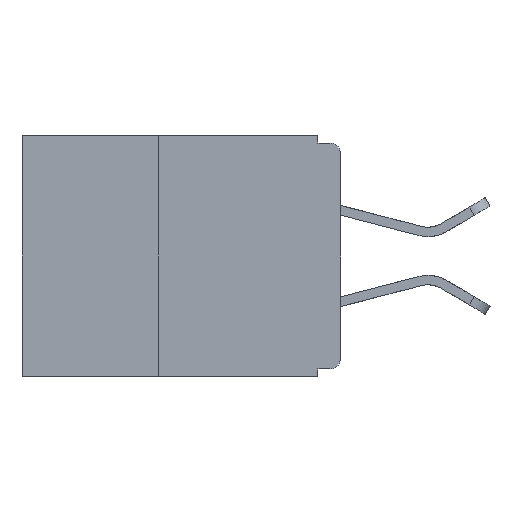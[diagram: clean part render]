
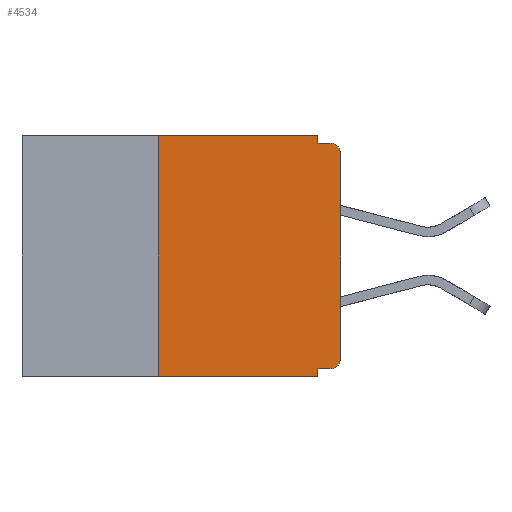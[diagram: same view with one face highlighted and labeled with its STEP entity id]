
A CAD part, left-side view. The second image highlights one B-rep face of the part: STEP entity #4534.
In plain terms, the highlighted planar face has unit normal (-1, 0, 0).
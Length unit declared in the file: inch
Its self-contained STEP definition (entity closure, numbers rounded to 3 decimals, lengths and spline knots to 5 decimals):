
#111 = CARTESIAN_POINT ( 'NONE',  ( 0., 0.031, 0. ) ) ;
#301 = CARTESIAN_POINT ( 'NONE',  ( 0., 0., -0.32 ) ) ;
#302 = CARTESIAN_POINT ( 'NONE',  ( 0., 0., -0.025 ) ) ;
#373 = DIRECTION ( 'NONE',  ( 0., 1., 0. ) ) ;
#602 = DIRECTION ( 'NONE',  ( 0., 0., -1. ) ) ;
#776 = VERTEX_POINT ( 'NONE', #18537 ) ;
#966 = CARTESIAN_POINT ( 'NONE',  ( 0., 0.031, -0.33 ) ) ;
#1257 = DIRECTION ( 'NONE',  ( -1., 0., 0. ) ) ;
#1378 = EDGE_LOOP ( 'NONE', ( #11181, #12087, #12539, #12990, #17019, #17448, #14291, #17869, #10957, #3368 ) ) ;
#1664 = DIRECTION ( 'NONE',  ( 0., 0., -1. ) ) ;
#1683 = DIRECTION ( 'NONE',  ( -1., 0., 0. ) ) ;
#1689 = CARTESIAN_POINT ( 'NONE',  ( 0., 0.015, -0.025 ) ) ;
#1736 = AXIS2_PLACEMENT_3D ( 'NONE', #1835, #1257, #602 ) ;
#1835 = CARTESIAN_POINT ( 'NONE',  ( 0., 0.015, -0.305 ) ) ;
#2115 = VECTOR ( 'NONE', #15954, 39.37008 ) ;
#2539 = CARTESIAN_POINT ( 'NONE',  ( 0., 0.031, -0.32 ) ) ;
#2722 = VECTOR ( 'NONE', #5000, 39.37008 ) ;
#3055 = VERTEX_POINT ( 'NONE', #302 ) ;
#3368 = ORIENTED_EDGE ( 'NONE', *, *, #5415, .T. ) ;
#3526 = VECTOR ( 'NONE', #8269, 39.37008 ) ;
#3916 = VECTOR ( 'NONE', #11428, 39.37008 ) ;
#4034 = LINE ( 'NONE', #8231, #3526 ) ;
#4182 = AXIS2_PLACEMENT_3D ( 'NONE', #1689, #1683, #1664 ) ;
#4226 = CARTESIAN_POINT ( 'NONE',  ( 0., 0.015, -0.32 ) ) ;
#4534 = ADVANCED_FACE ( 'NONE', ( #9555 ), #14995, .F. ) ;
#4952 = CARTESIAN_POINT ( 'NONE',  ( 0., 0.437, -0.33 ) ) ;
#5000 = DIRECTION ( 'NONE',  ( 0., -1., 0. ) ) ;
#5022 = CARTESIAN_POINT ( 'NONE',  ( 0., 0., -0.01 ) ) ;
#5252 = VERTEX_POINT ( 'NONE', #111 ) ;
#5415 = EDGE_CURVE ( 'NONE', #12051, #15168, #18578, .T. ) ;
#5554 = CARTESIAN_POINT ( 'NONE',  ( 0., 0.25, -0.33 ) ) ;
#5567 = CARTESIAN_POINT ( 'NONE',  ( 0., 0., -0.305 ) ) ;
#5965 = CARTESIAN_POINT ( 'NONE',  ( 0., 0.031, 0. ) ) ;
#6213 = VECTOR ( 'NONE', #6571, 39.37008 ) ;
#6506 = VERTEX_POINT ( 'NONE', #966 ) ;
#6571 = DIRECTION ( 'NONE',  ( 0., -1., 0. ) ) ;
#6614 = LINE ( 'NONE', #16794, #17921 ) ;
#6854 = LINE ( 'NONE', #4952, #2722 ) ;
#8231 = CARTESIAN_POINT ( 'NONE',  ( 0., 0.031, -0.33 ) ) ;
#8269 = DIRECTION ( 'NONE',  ( 0., 0., -1. ) ) ;
#8357 = VERTEX_POINT ( 'NONE', #2539 ) ;
#8415 = EDGE_CURVE ( 'NONE', #3055, #16793, #11207, .T. ) ;
#9001 = VERTEX_POINT ( 'NONE', #10306 ) ;
#9039 = EDGE_CURVE ( 'NONE', #15168, #3055, #18685, .T. ) ;
#9431 = CARTESIAN_POINT ( 'NONE',  ( 0., 0., 0. ) ) ;
#9555 = FACE_OUTER_BOUND ( 'NONE', #1378, .T. ) ;
#10234 = LINE ( 'NONE', #5965, #2115 ) ;
#10306 = CARTESIAN_POINT ( 'NONE',  ( 0., 0.25, 0. ) ) ;
#10372 = DIRECTION ( 'NONE',  ( 0., 0., 1. ) ) ;
#10957 = ORIENTED_EDGE ( 'NONE', *, *, #11390, .F. ) ;
#11181 = ORIENTED_EDGE ( 'NONE', *, *, #9039, .T. ) ;
#11207 = CIRCLE ( 'NONE', #4182, 0.015 ) ;
#11390 = EDGE_CURVE ( 'NONE', #12051, #8357, #18850, .T. ) ;
#11428 = DIRECTION ( 'NONE',  ( 0., -1., 0. ) ) ;
#11862 = EDGE_CURVE ( 'NONE', #8357, #6506, #4034, .T. ) ;
#11908 = LINE ( 'NONE', #12014, #3916 ) ;
#12014 = CARTESIAN_POINT ( 'NONE',  ( 0., 0.437, 0. ) ) ;
#12051 = VERTEX_POINT ( 'NONE', #4226 ) ;
#12087 = ORIENTED_EDGE ( 'NONE', *, *, #8415, .T. ) ;
#12539 = ORIENTED_EDGE ( 'NONE', *, *, #17848, .F. ) ;
#12990 = ORIENTED_EDGE ( 'NONE', *, *, #16503, .F. ) ;
#13776 = EDGE_CURVE ( 'NONE', #18763, #6506, #6854, .T. ) ;
#14291 = ORIENTED_EDGE ( 'NONE', *, *, #13776, .T. ) ;
#14353 = EDGE_CURVE ( 'NONE', #9001, #5252, #11908, .T. ) ;
#14674 = EDGE_CURVE ( 'NONE', #18763, #9001, #6614, .T. ) ;
#14897 = DIRECTION ( 'NONE',  ( 0., 0., -1. ) ) ;
#14941 = DIRECTION ( 'NONE',  ( 1., 0., 0. ) ) ;
#14995 = PLANE ( 'NONE',  #18531 ) ;
#15168 = VERTEX_POINT ( 'NONE', #5567 ) ;
#15276 = VECTOR ( 'NONE', #373, 39.37008 ) ;
#15346 = CARTESIAN_POINT ( 'NONE',  ( 0., 0.015, -0.01 ) ) ;
#15526 = CARTESIAN_POINT ( 'NONE',  ( 0., 0.437, 0. ) ) ;
#15954 = DIRECTION ( 'NONE',  ( 0., 0., -1. ) ) ;
#16503 = EDGE_CURVE ( 'NONE', #5252, #776, #10234, .T. ) ;
#16793 = VERTEX_POINT ( 'NONE', #15346 ) ;
#16794 = CARTESIAN_POINT ( 'NONE',  ( 0., 0.25, -0.33 ) ) ;
#17019 = ORIENTED_EDGE ( 'NONE', *, *, #14353, .F. ) ;
#17051 = DIRECTION ( 'NONE',  ( 0., 0., 1. ) ) ;
#17448 = ORIENTED_EDGE ( 'NONE', *, *, #14674, .F. ) ;
#17561 = LINE ( 'NONE', #5022, #6213 ) ;
#17848 = EDGE_CURVE ( 'NONE', #776, #16793, #17561, .T. ) ;
#17869 = ORIENTED_EDGE ( 'NONE', *, *, #11862, .F. ) ;
#17921 = VECTOR ( 'NONE', #17051, 39.37008 ) ;
#18256 = VECTOR ( 'NONE', #10372, 39.37008 ) ;
#18531 = AXIS2_PLACEMENT_3D ( 'NONE', #15526, #14941, #14897 ) ;
#18537 = CARTESIAN_POINT ( 'NONE',  ( 0., 0.031, -0.01 ) ) ;
#18578 = CIRCLE ( 'NONE', #1736, 0.015 ) ;
#18685 = LINE ( 'NONE', #9431, #18256 ) ;
#18763 = VERTEX_POINT ( 'NONE', #5554 ) ;
#18850 = LINE ( 'NONE', #301, #15276 ) ;
